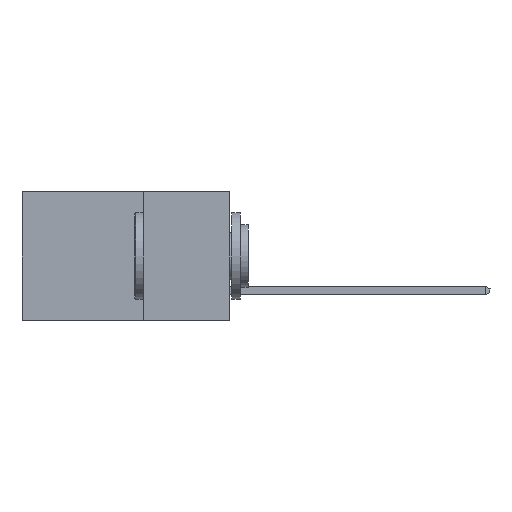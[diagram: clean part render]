
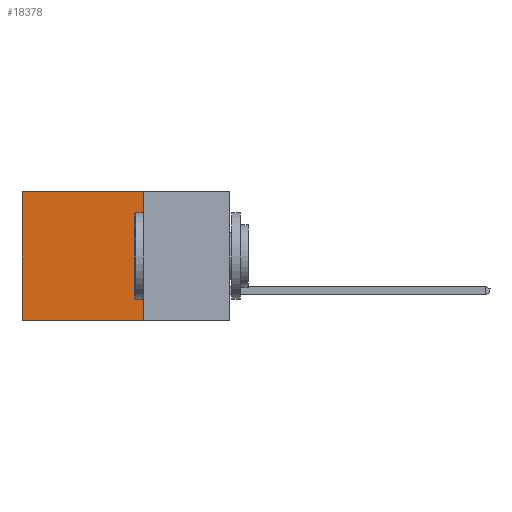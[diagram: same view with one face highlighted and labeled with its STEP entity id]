
A CAD part, left-side view. The second image highlights one B-rep face of the part: STEP entity #18378.
In plain terms, the highlighted planar face has unit normal (-1, 0, 0).
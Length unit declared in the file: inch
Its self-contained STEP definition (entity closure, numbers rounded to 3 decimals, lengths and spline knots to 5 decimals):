
#183 = VECTOR ( 'NONE', #19356, 39.37008 ) ;
#2598 = LINE ( 'NONE', #4408, #16478 ) ;
#2745 = VECTOR ( 'NONE', #18019, 39.37008 ) ;
#3027 = CARTESIAN_POINT ( 'NONE',  ( 0.2615, 0.6, -0.37 ) ) ;
#3284 = CARTESIAN_POINT ( 'NONE',  ( 0.2615, 0.6, -0.37 ) ) ;
#4408 = CARTESIAN_POINT ( 'NONE',  ( 0.2615, 0.25, 0. ) ) ;
#4734 = VECTOR ( 'NONE', #7160, 39.37008 ) ;
#4770 = PLANE ( 'NONE',  #24461 ) ;
#5374 = CARTESIAN_POINT ( 'NONE',  ( 0.2615, 0.25, -0.37 ) ) ;
#6889 = EDGE_CURVE ( 'NONE', #17859, #24843, #24620, .T. ) ;
#7160 = DIRECTION ( 'NONE',  ( 0., 0., -1. ) ) ;
#7557 = ORIENTED_EDGE ( 'NONE', *, *, #19636, .F. ) ;
#8741 = DIRECTION ( 'NONE',  ( 1., 0., 0. ) ) ;
#10178 = DIRECTION ( 'NONE',  ( 0., 1., 0. ) ) ;
#10784 = DIRECTION ( 'NONE',  ( 0., 0., -1. ) ) ;
#11021 = ORIENTED_EDGE ( 'NONE', *, *, #11915, .T. ) ;
#11915 = EDGE_CURVE ( 'NONE', #20114, #17859, #2598, .T. ) ;
#12366 = CARTESIAN_POINT ( 'NONE',  ( 0.2615, 0.6, 0. ) ) ;
#13435 = CARTESIAN_POINT ( 'NONE',  ( 0.2615, 0.25, -0.37 ) ) ;
#13780 = ORIENTED_EDGE ( 'NONE', *, *, #14934, .F. ) ;
#14272 = LINE ( 'NONE', #17771, #2745 ) ;
#14326 = ORIENTED_EDGE ( 'NONE', *, *, #6889, .T. ) ;
#14934 = EDGE_CURVE ( 'NONE', #21677, #24843, #15629, .T. ) ;
#15629 = LINE ( 'NONE', #13435, #183 ) ;
#16478 = VECTOR ( 'NONE', #10178, 39.37008 ) ;
#17771 = CARTESIAN_POINT ( 'NONE',  ( 0.2615, 0.25, -0.37 ) ) ;
#17859 = VERTEX_POINT ( 'NONE', #12366 ) ;
#18019 = DIRECTION ( 'NONE',  ( 0., 0., -1. ) ) ;
#18378 = ADVANCED_FACE ( 'NONE', ( #22619 ), #4770, .F. ) ;
#19356 = DIRECTION ( 'NONE',  ( 0., 1., 0. ) ) ;
#19636 = EDGE_CURVE ( 'NONE', #20114, #21677, #14272, .T. ) ;
#20114 = VERTEX_POINT ( 'NONE', #24023 ) ;
#20334 = CARTESIAN_POINT ( 'NONE',  ( 0.2615, 0.25, -0.37 ) ) ;
#21677 = VERTEX_POINT ( 'NONE', #5374 ) ;
#22619 = FACE_OUTER_BOUND ( 'NONE', #25156, .T. ) ;
#24023 = CARTESIAN_POINT ( 'NONE',  ( 0.2615, 0.25, 0. ) ) ;
#24461 = AXIS2_PLACEMENT_3D ( 'NONE', #20334, #8741, #10784 ) ;
#24620 = LINE ( 'NONE', #3284, #4734 ) ;
#24843 = VERTEX_POINT ( 'NONE', #3027 ) ;
#25156 = EDGE_LOOP ( 'NONE', ( #14326, #13780, #7557, #11021 ) ) ;
